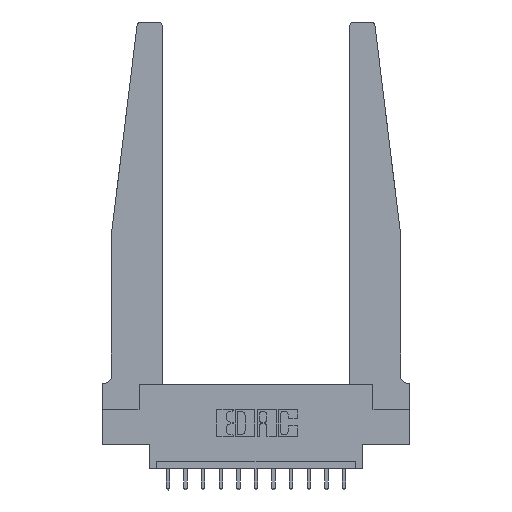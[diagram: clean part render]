
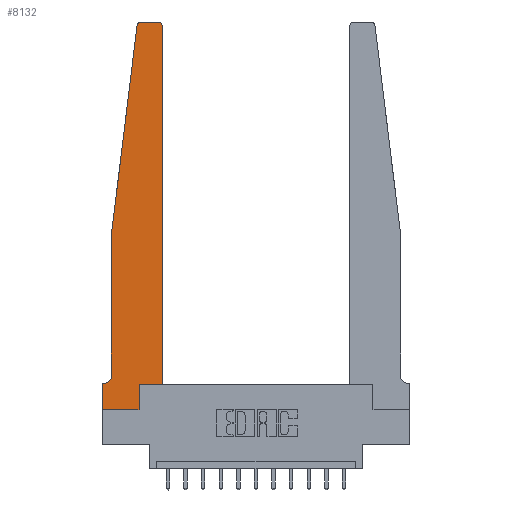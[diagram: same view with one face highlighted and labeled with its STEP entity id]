
A CAD part, top view. The second image highlights one B-rep face of the part: STEP entity #8132.
In plain terms, the highlighted planar face has unit normal (0, 0, 1).
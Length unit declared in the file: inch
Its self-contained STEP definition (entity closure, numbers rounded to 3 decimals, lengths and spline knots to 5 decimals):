
#138 = VERTEX_POINT ( 'NONE', #10795 ) ;
#234 = VECTOR ( 'NONE', #6549, 39.37008 ) ;
#457 = LINE ( 'NONE', #13701, #12784 ) ;
#658 = EDGE_CURVE ( 'NONE', #6288, #12103, #8652, .T. ) ;
#942 = DIRECTION ( 'NONE',  ( 0., 0., 1. ) ) ;
#1023 = VERTEX_POINT ( 'NONE', #5056 ) ;
#1461 = CARTESIAN_POINT ( 'NONE',  ( 0.065, 0.2375, 0.37 ) ) ;
#1584 = DIRECTION ( 'NONE',  ( 0., 1., 0. ) ) ;
#1656 = CARTESIAN_POINT ( 'NONE',  ( 0.24675, 2.72367, 0.37 ) ) ;
#1692 = DIRECTION ( 'NONE',  ( 1., 0., 0. ) ) ;
#1893 = VERTEX_POINT ( 'NONE', #7081 ) ;
#2000 = CIRCLE ( 'NONE', #4601, 0.05 ) ;
#2810 = ORIENTED_EDGE ( 'NONE', *, *, #4172, .T. ) ;
#2950 = DIRECTION ( 'NONE',  ( 0., 0., -1. ) ) ;
#2969 = VERTEX_POINT ( 'NONE', #12374 ) ;
#3140 = VECTOR ( 'NONE', #9033, 39.37008 ) ;
#3301 = DIRECTION ( 'NONE',  ( 0., 0., 1. ) ) ;
#3492 = LINE ( 'NONE', #15244, #234 ) ;
#3600 = VERTEX_POINT ( 'NONE', #5303 ) ;
#4148 = LINE ( 'NONE', #6622, #15657 ) ;
#4172 = EDGE_CURVE ( 'NONE', #8708, #14955, #4148, .T. ) ;
#4524 = EDGE_CURVE ( 'NONE', #3600, #2969, #12580, .T. ) ;
#4601 = AXIS2_PLACEMENT_3D ( 'NONE', #5583, #2950, #10452 ) ;
#4860 = DIRECTION ( 'NONE',  ( -1., 0., 0. ) ) ;
#5056 = CARTESIAN_POINT ( 'NONE',  ( 0.395, 2.75, 0.37 ) ) ;
#5303 = CARTESIAN_POINT ( 'NONE',  ( 0.015, 0.1875, 0.37 ) ) ;
#5306 = CARTESIAN_POINT ( 'NONE',  ( 0.065, 1.25, 0.37 ) ) ;
#5320 = LINE ( 'NONE', #13773, #8014 ) ;
#5441 = CARTESIAN_POINT ( 'NONE',  ( 0., 0., 0.37 ) ) ;
#5583 = CARTESIAN_POINT ( 'NONE',  ( 0.015, 0.2375, 0.37 ) ) ;
#5875 = CARTESIAN_POINT ( 'NONE',  ( 0.395, 2.72, 0.37 ) ) ;
#5981 = CARTESIAN_POINT ( 'NONE',  ( 0.27653, 2.72, 0.37 ) ) ;
#6019 = ORIENTED_EDGE ( 'NONE', *, *, #13722, .T. ) ;
#6196 = LINE ( 'NONE', #8816, #11754 ) ;
#6253 = DIRECTION ( 'NONE',  ( 0., 1., 0. ) ) ;
#6288 = VERTEX_POINT ( 'NONE', #13291 ) ;
#6389 = ORIENTED_EDGE ( 'NONE', *, *, #15736, .T. ) ;
#6390 = CARTESIAN_POINT ( 'NONE',  ( 0.425, 0.18, 0.37 ) ) ;
#6549 = DIRECTION ( 'NONE',  ( 1., 0., 0. ) ) ;
#6622 = CARTESIAN_POINT ( 'NONE',  ( 0.065, 1.25, 0.37 ) ) ;
#6652 = EDGE_LOOP ( 'NONE', ( #6019, #12349, #14473, #2810, #13561, #10843, #6389, #11906, #12376, #11597, #12408, #7172 ) ) ;
#6963 = CARTESIAN_POINT ( 'NONE',  ( 0., 0., 0.37 ) ) ;
#7033 = EDGE_CURVE ( 'NONE', #12103, #1023, #8471, .T. ) ;
#7081 = CARTESIAN_POINT ( 'NONE',  ( 0.27653, 2.75, 0.37 ) ) ;
#7172 = ORIENTED_EDGE ( 'NONE', *, *, #7033, .T. ) ;
#7820 = VERTEX_POINT ( 'NONE', #1656 ) ;
#7937 = CARTESIAN_POINT ( 'NONE',  ( 0., 0.1875, 0.37 ) ) ;
#8014 = VECTOR ( 'NONE', #9025, 39.37008 ) ;
#8132 = ADVANCED_FACE ( 'NONE', ( #11704 ), #11631, .T. ) ;
#8135 = EDGE_CURVE ( 'NONE', #12459, #13928, #12880, .T. ) ;
#8462 = VECTOR ( 'NONE', #1584, 39.37008 ) ;
#8471 = CIRCLE ( 'NONE', #15786, 0.03 ) ;
#8606 = CARTESIAN_POINT ( 'NONE',  ( 0.25, 2.75, 0.37 ) ) ;
#8652 = LINE ( 'NONE', #6390, #8462 ) ;
#8708 = VERTEX_POINT ( 'NONE', #5306 ) ;
#8816 = CARTESIAN_POINT ( 'NONE',  ( 0., 0., 0.37 ) ) ;
#8887 = CIRCLE ( 'NONE', #15178, 0.03 ) ;
#9025 = DIRECTION ( 'NONE',  ( -0.122, -0.992, 0. ) ) ;
#9033 = DIRECTION ( 'NONE',  ( -1., 0., 0. ) ) ;
#9044 = VECTOR ( 'NONE', #12935, 39.37008 ) ;
#9717 = VECTOR ( 'NONE', #4860, 39.37008 ) ;
#10452 = DIRECTION ( 'NONE',  ( -1., 0., 0. ) ) ;
#10691 = DIRECTION ( 'NONE',  ( 1., 0., 0. ) ) ;
#10795 = CARTESIAN_POINT ( 'NONE',  ( 0.2605, 0.18, 0.37 ) ) ;
#10843 = ORIENTED_EDGE ( 'NONE', *, *, #4524, .T. ) ;
#11597 = ORIENTED_EDGE ( 'NONE', *, *, #12219, .T. ) ;
#11631 = PLANE ( 'NONE',  #14401 ) ;
#11704 = FACE_OUTER_BOUND ( 'NONE', #6652, .T. ) ;
#11754 = VECTOR ( 'NONE', #15084, 39.37008 ) ;
#11906 = ORIENTED_EDGE ( 'NONE', *, *, #8135, .T. ) ;
#12103 = VERTEX_POINT ( 'NONE', #14816 ) ;
#12219 = EDGE_CURVE ( 'NONE', #138, #6288, #3492, .T. ) ;
#12349 = ORIENTED_EDGE ( 'NONE', *, *, #12898, .T. ) ;
#12374 = CARTESIAN_POINT ( 'NONE',  ( 0., 0.1875, 0.37 ) ) ;
#12376 = ORIENTED_EDGE ( 'NONE', *, *, #14134, .T. ) ;
#12408 = ORIENTED_EDGE ( 'NONE', *, *, #658, .T. ) ;
#12459 = VERTEX_POINT ( 'NONE', #6963 ) ;
#12580 = LINE ( 'NONE', #15245, #3140 ) ;
#12784 = VECTOR ( 'NONE', #6253, 39.37008 ) ;
#12880 = LINE ( 'NONE', #5441, #9044 ) ;
#12898 = EDGE_CURVE ( 'NONE', #1893, #7820, #8887, .T. ) ;
#12935 = DIRECTION ( 'NONE',  ( 1., 0., 0. ) ) ;
#13291 = CARTESIAN_POINT ( 'NONE',  ( 0.425, 0.18, 0.37 ) ) ;
#13561 = ORIENTED_EDGE ( 'NONE', *, *, #13910, .T. ) ;
#13701 = CARTESIAN_POINT ( 'NONE',  ( 0.2605, 0.18, 0.37 ) ) ;
#13722 = EDGE_CURVE ( 'NONE', #1023, #1893, #15303, .T. ) ;
#13773 = CARTESIAN_POINT ( 'NONE',  ( 0.065, 1.25, 0.37 ) ) ;
#13847 = EDGE_CURVE ( 'NONE', #7820, #8708, #5320, .T. ) ;
#13910 = EDGE_CURVE ( 'NONE', #14955, #3600, #2000, .T. ) ;
#13928 = VERTEX_POINT ( 'NONE', #14055 ) ;
#14055 = CARTESIAN_POINT ( 'NONE',  ( 0.2605, 0., 0.37 ) ) ;
#14134 = EDGE_CURVE ( 'NONE', #13928, #138, #457, .T. ) ;
#14401 = AXIS2_PLACEMENT_3D ( 'NONE', #7937, #15304, #1692 ) ;
#14473 = ORIENTED_EDGE ( 'NONE', *, *, #13847, .T. ) ;
#14816 = CARTESIAN_POINT ( 'NONE',  ( 0.425, 2.72, 0.37 ) ) ;
#14955 = VERTEX_POINT ( 'NONE', #1461 ) ;
#15084 = DIRECTION ( 'NONE',  ( 0., -1., 0. ) ) ;
#15178 = AXIS2_PLACEMENT_3D ( 'NONE', #5981, #3301, #10691 ) ;
#15202 = DIRECTION ( 'NONE',  ( 0., -1., 0. ) ) ;
#15244 = CARTESIAN_POINT ( 'NONE',  ( 0.425, 0.18, 0.37 ) ) ;
#15245 = CARTESIAN_POINT ( 'NONE',  ( 0.065, 0.1875, 0.37 ) ) ;
#15303 = LINE ( 'NONE', #8606, #9717 ) ;
#15304 = DIRECTION ( 'NONE',  ( 0., 0., 1. ) ) ;
#15657 = VECTOR ( 'NONE', #15202, 39.37008 ) ;
#15677 = DIRECTION ( 'NONE',  ( 1., 0., 0. ) ) ;
#15736 = EDGE_CURVE ( 'NONE', #2969, #12459, #6196, .T. ) ;
#15786 = AXIS2_PLACEMENT_3D ( 'NONE', #5875, #942, #15677 ) ;
